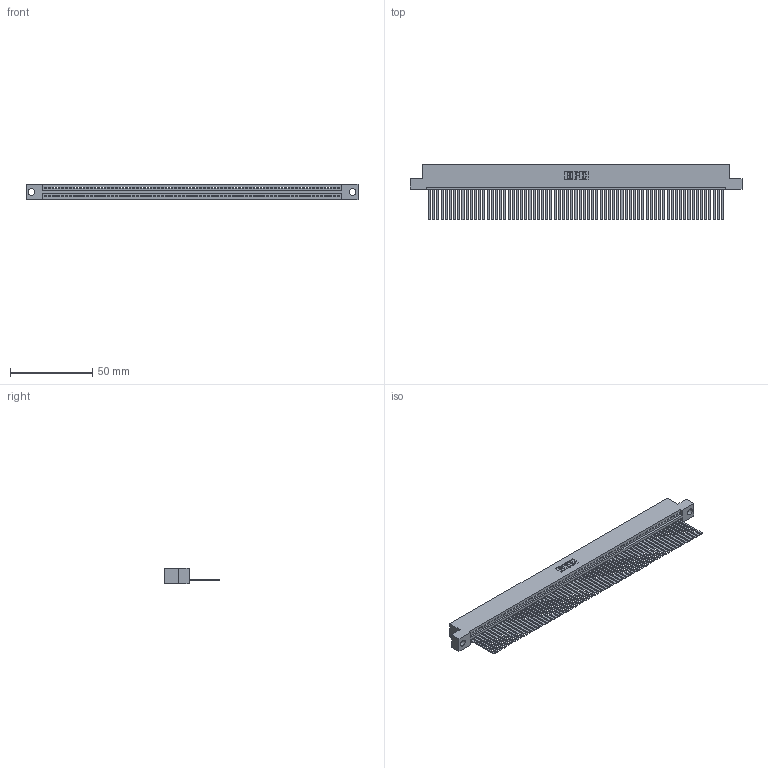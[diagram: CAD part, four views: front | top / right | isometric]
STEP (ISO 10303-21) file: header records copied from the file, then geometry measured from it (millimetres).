
FILE_DESCRIPTION (( 'STEP AP203' ), '1' );
FILE_NAME ('345-071-544-104.STEP', '2018-10-01T15:48:01', ( '' ), ( '' ), 'SwSTEP 2.0', 'SolidWorks 2016', '' );
FILE_SCHEMA (( 'CONFIG_CONTROL_DESIGN' ));
Length unit declared in the file: inch
Products named in the file (3): 345 Part_Flush Mounting Lugs - 0.156 Dia-TH; 345-071-544-104; 345-292-001_345-293-144
Assembly tree (72 placements, depth 2):
  345-071-544-104
    345 Part_Flush Mounting Lugs - 0.156 Dia-TH
    345-292-001_345-293-144  x71
Bounding box: 201.55 x 33.96 x 9.4 mm (x, y, z)
Volume: 20115.3 mm3; surface area: 29402.9 mm2
Topology: 72 solids, 72 shells, 3818 faces, 11559 edges, 7610 vertices
Faces by surface type: plane 2636, cylinder 1182
Entity records: 49351 total; most frequent: ORIENTED_EDGE 8558, CARTESIAN_POINT 8553, DIRECTION 7425, EDGE_CURVE 4279, VECTOR 3867, LINE 3867, VERTEX_POINT 2850, AXIS2_PLACEMENT_3D 1779
